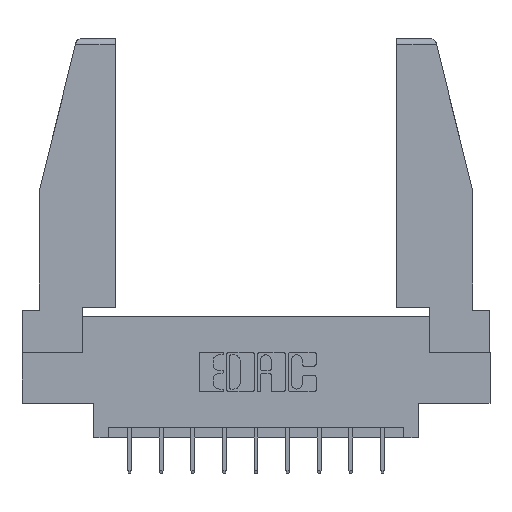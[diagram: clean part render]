
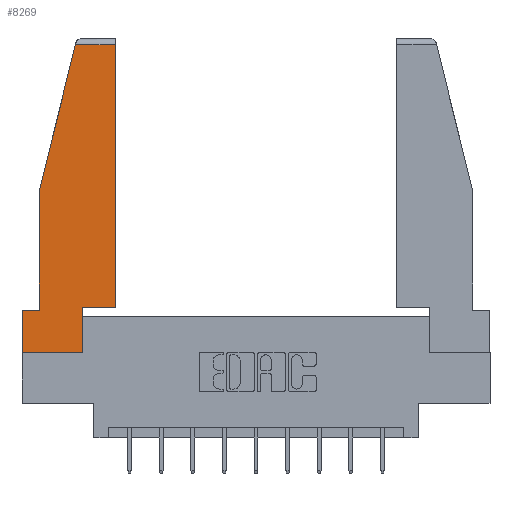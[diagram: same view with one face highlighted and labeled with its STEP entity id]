
A CAD part, top view. The second image highlights one B-rep face of the part: STEP entity #8269.
In plain terms, the highlighted planar face has unit normal (0, 0, 1).
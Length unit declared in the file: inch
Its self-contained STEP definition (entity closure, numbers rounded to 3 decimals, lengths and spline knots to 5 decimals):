
#4 = CARTESIAN_POINT ( 'NONE',  ( 0.086, 0.8, 0. ) ) ;
#42 = EDGE_CURVE ( 'NONE', #7624, #12013, #12521, .T. ) ;
#391 = ORIENTED_EDGE ( 'NONE', *, *, #11708, .T. ) ;
#557 = CARTESIAN_POINT ( 'NONE',  ( 0., 0.21, 0. ) ) ;
#759 = PLANE ( 'NONE',  #12742 ) ;
#1126 = ORIENTED_EDGE ( 'NONE', *, *, #8577, .T. ) ;
#1264 = ORIENTED_EDGE ( 'NONE', *, *, #5259, .T. ) ;
#1353 = VECTOR ( 'NONE', #12011, 39.37008 ) ;
#1663 = DIRECTION ( 'NONE',  ( 1., 0., 0. ) ) ;
#1726 = DIRECTION ( 'NONE',  ( 0., -1., 0. ) ) ;
#2429 = LINE ( 'NONE', #13037, #4254 ) ;
#2439 = FACE_OUTER_BOUND ( 'NONE', #4666, .T. ) ;
#2499 = CARTESIAN_POINT ( 'NONE',  ( 0.297, 0., 0. ) ) ;
#2775 = DIRECTION ( 'NONE',  ( -1., 0., 0. ) ) ;
#2844 = LINE ( 'NONE', #13289, #5049 ) ;
#2897 = EDGE_CURVE ( 'NONE', #13340, #12473, #5054, .T. ) ;
#3127 = LINE ( 'NONE', #7883, #8541 ) ;
#3133 = DIRECTION ( 'NONE',  ( 1., 0., 0. ) ) ;
#3217 = ORIENTED_EDGE ( 'NONE', *, *, #2897, .T. ) ;
#3243 = EDGE_CURVE ( 'NONE', #8824, #9080, #6415, .T. ) ;
#3298 = ORIENTED_EDGE ( 'NONE', *, *, #7283, .T. ) ;
#3363 = VECTOR ( 'NONE', #9810, 39.37008 ) ;
#3512 = DIRECTION ( 'NONE',  ( -0.239, -0.971, 0. ) ) ;
#3672 = ORIENTED_EDGE ( 'NONE', *, *, #3243, .T. ) ;
#4254 = VECTOR ( 'NONE', #9831, 39.37008 ) ;
#4666 = EDGE_LOOP ( 'NONE', ( #391, #12999, #3298, #3672, #1126, #1264, #3217, #10179, #10465 ) ) ;
#4944 = EDGE_CURVE ( 'NONE', #13917, #9083, #8116, .T. ) ;
#5049 = VECTOR ( 'NONE', #9034, 39.37008 ) ;
#5054 = LINE ( 'NONE', #10599, #9101 ) ;
#5084 = DIRECTION ( 'NONE',  ( 0., 0., 1. ) ) ;
#5259 = EDGE_CURVE ( 'NONE', #13884, #13340, #2844, .T. ) ;
#5303 = VECTOR ( 'NONE', #10767, 39.37008 ) ;
#5473 = CARTESIAN_POINT ( 'NONE',  ( 0.086, 0.21, 0. ) ) ;
#5602 = CARTESIAN_POINT ( 'NONE',  ( 0., 1.52, 0. ) ) ;
#5741 = VECTOR ( 'NONE', #1726, 39.37008 ) ;
#5966 = CARTESIAN_POINT ( 'NONE',  ( 0., 0.21, 0. ) ) ;
#6415 = LINE ( 'NONE', #8379, #5741 ) ;
#7283 = EDGE_CURVE ( 'NONE', #9083, #8824, #3127, .T. ) ;
#7624 = VERTEX_POINT ( 'NONE', #12567 ) ;
#7883 = CARTESIAN_POINT ( 'NONE',  ( 0.271, 1.55, 0. ) ) ;
#8116 = LINE ( 'NONE', #5602, #1353 ) ;
#8269 = ADVANCED_FACE ( 'NONE', ( #2439 ), #759, .T. ) ;
#8379 = CARTESIAN_POINT ( 'NONE',  ( 0.086, 0.8, 0. ) ) ;
#8541 = VECTOR ( 'NONE', #3512, 39.37008 ) ;
#8577 = EDGE_CURVE ( 'NONE', #9080, #13884, #13512, .T. ) ;
#8824 = VERTEX_POINT ( 'NONE', #4 ) ;
#9034 = DIRECTION ( 'NONE',  ( 0., -1., 0. ) ) ;
#9080 = VERTEX_POINT ( 'NONE', #5473 ) ;
#9083 = VERTEX_POINT ( 'NONE', #12895 ) ;
#9101 = VECTOR ( 'NONE', #3133, 39.37008 ) ;
#9365 = CARTESIAN_POINT ( 'NONE',  ( 0., 0., 0. ) ) ;
#9455 = EDGE_CURVE ( 'NONE', #12473, #7624, #2429, .T. ) ;
#9810 = DIRECTION ( 'NONE',  ( 0., 1., 0. ) ) ;
#9831 = DIRECTION ( 'NONE',  ( 0., 1., 0. ) ) ;
#10095 = LINE ( 'NONE', #12883, #3363 ) ;
#10179 = ORIENTED_EDGE ( 'NONE', *, *, #9455, .T. ) ;
#10307 = VECTOR ( 'NONE', #2775, 39.37008 ) ;
#10465 = ORIENTED_EDGE ( 'NONE', *, *, #42, .T. ) ;
#10599 = CARTESIAN_POINT ( 'NONE',  ( 0., 0., 0. ) ) ;
#10767 = DIRECTION ( 'NONE',  ( 1., 0., 0. ) ) ;
#11355 = CARTESIAN_POINT ( 'NONE',  ( 0.461, 0.223, 0. ) ) ;
#11708 = EDGE_CURVE ( 'NONE', #12013, #13917, #10095, .T. ) ;
#11859 = CARTESIAN_POINT ( 'NONE',  ( 0.297, 0.223, 0. ) ) ;
#12011 = DIRECTION ( 'NONE',  ( -1., 0., 0. ) ) ;
#12013 = VERTEX_POINT ( 'NONE', #11355 ) ;
#12390 = CARTESIAN_POINT ( 'NONE',  ( 0.461, 1.52, 0. ) ) ;
#12473 = VERTEX_POINT ( 'NONE', #2499 ) ;
#12521 = LINE ( 'NONE', #11859, #5303 ) ;
#12567 = CARTESIAN_POINT ( 'NONE',  ( 0.297, 0.223, 0. ) ) ;
#12742 = AXIS2_PLACEMENT_3D ( 'NONE', #9365, #5084, #1663 ) ;
#12883 = CARTESIAN_POINT ( 'NONE',  ( 0.461, 0.223, 0. ) ) ;
#12895 = CARTESIAN_POINT ( 'NONE',  ( 0.2636, 1.52, 0. ) ) ;
#12999 = ORIENTED_EDGE ( 'NONE', *, *, #4944, .T. ) ;
#13037 = CARTESIAN_POINT ( 'NONE',  ( 0.297, 0., 0. ) ) ;
#13289 = CARTESIAN_POINT ( 'NONE',  ( 0., 0.21, 0. ) ) ;
#13340 = VERTEX_POINT ( 'NONE', #13710 ) ;
#13512 = LINE ( 'NONE', #5966, #10307 ) ;
#13710 = CARTESIAN_POINT ( 'NONE',  ( 0., 0., 0. ) ) ;
#13884 = VERTEX_POINT ( 'NONE', #557 ) ;
#13917 = VERTEX_POINT ( 'NONE', #12390 ) ;
